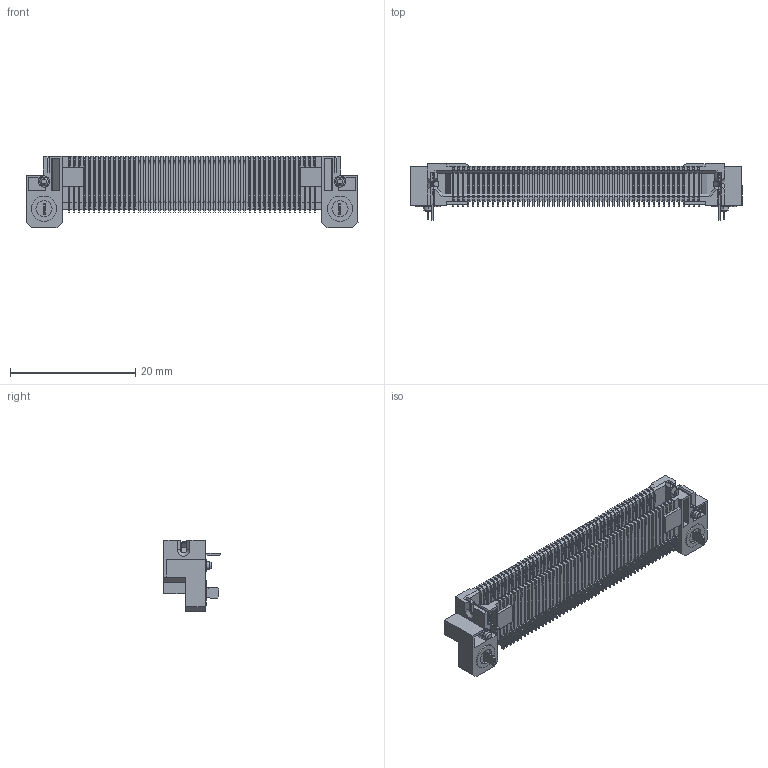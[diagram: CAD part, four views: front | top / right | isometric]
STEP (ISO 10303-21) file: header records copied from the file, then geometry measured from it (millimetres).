
FILE_DESCRIPTION (( 'STEP AP214' ), '1' );
FILE_NAME ('473-100-571-002.STEP', '2020-05-20T19:04:57', ( '' ), ( '' ), 'SwSTEP 2.0', 'SolidWorks 2020', '' );
FILE_SCHEMA (( 'AUTOMOTIVE_DESIGN' ));
Length unit declared in the file: millimetre
Products named in the file (6): 473 Latch RH; 473-100-571-002 CON; 473-100-571-002 INS; 473-100-571-002 BM; 473 Latch LH; 473-100-571-002
Assembly tree (55 placements, depth 2):
  473-100-571-002
    473-100-571-002 INS
    473-100-571-002 CON  x50
    473-100-571-002 BM  x2
    473 Latch LH
    473 Latch RH
Bounding box: 53 x 9.02 x 11.35 mm (x, y, z)
Volume: 1486.4 mm3; surface area: 7019.1 mm2
Topology: 105 solids, 105 shells, 4395 faces, 12356 edges, 8178 vertices
Faces by surface type: plane 3584, cylinder 804, cone 7
Entity records: 71293 total; most frequent: CARTESIAN_POINT 12713, ORIENTED_EDGE 12608, DIRECTION 11472, EDGE_CURVE 6304, VECTOR 5590, LINE 5590, VERTEX_POINT 4144, AXIS2_PLACEMENT_3D 2941
